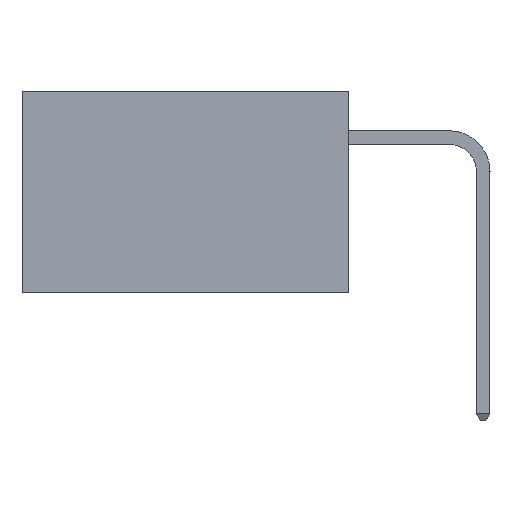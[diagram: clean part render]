
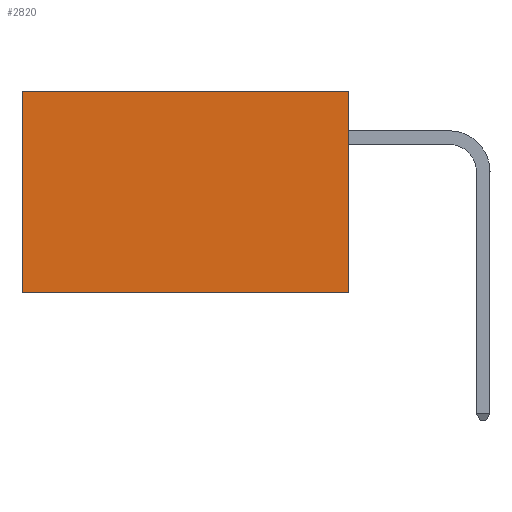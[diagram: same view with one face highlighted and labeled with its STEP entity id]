
A CAD part, left-side view. The second image highlights one B-rep face of the part: STEP entity #2820.
In plain terms, the highlighted planar face has unit normal (-1, 0, 0).
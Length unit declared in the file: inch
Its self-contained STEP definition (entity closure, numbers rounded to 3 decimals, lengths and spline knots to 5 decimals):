
#102 = DIRECTION ( 'NONE',  ( 0., 0., -1. ) ) ;
#106 = DIRECTION ( 'NONE',  ( 1., 0., 0. ) ) ;
#132 = CARTESIAN_POINT ( 'NONE',  ( 0.2875, 0., 0. ) ) ;
#206 = PLANE ( 'NONE',  #11907 ) ;
#261 = ORIENTED_EDGE ( 'NONE', *, *, #8044, .F. ) ;
#651 = CARTESIAN_POINT ( 'NONE',  ( 0.2875, 0., -0.37 ) ) ;
#794 = VECTOR ( 'NONE', #5014, 39.37008 ) ;
#1060 = CARTESIAN_POINT ( 'NONE',  ( 0.2875, 0., 0. ) ) ;
#1378 = CARTESIAN_POINT ( 'NONE',  ( 0.2875, 0., 0. ) ) ;
#1507 = ORIENTED_EDGE ( 'NONE', *, *, #5103, .F. ) ;
#2678 = LINE ( 'NONE', #10681, #14231 ) ;
#2820 = ADVANCED_FACE ( 'NONE', ( #4681 ), #206, .F. ) ;
#4428 = LINE ( 'NONE', #651, #794 ) ;
#4652 = VERTEX_POINT ( 'NONE', #6866 ) ;
#4681 = FACE_OUTER_BOUND ( 'NONE', #7970, .T. ) ;
#4703 = CARTESIAN_POINT ( 'NONE',  ( 0.2875, 0.6, -0.37 ) ) ;
#5014 = DIRECTION ( 'NONE',  ( 0., 1., 0. ) ) ;
#5103 = EDGE_CURVE ( 'NONE', #10782, #11506, #4428, .T. ) ;
#5177 = DIRECTION ( 'NONE',  ( 0., 0., -1. ) ) ;
#5196 = VERTEX_POINT ( 'NONE', #1060 ) ;
#6180 = DIRECTION ( 'NONE',  ( 0., 1., 0. ) ) ;
#6442 = DIRECTION ( 'NONE',  ( 0., 0., -1. ) ) ;
#6866 = CARTESIAN_POINT ( 'NONE',  ( 0.2875, 0.6, 0. ) ) ;
#7374 = ORIENTED_EDGE ( 'NONE', *, *, #10462, .T. ) ;
#7970 = EDGE_LOOP ( 'NONE', ( #11912, #1507, #261, #7374 ) ) ;
#8044 = EDGE_CURVE ( 'NONE', #5196, #10782, #2678, .T. ) ;
#8862 = VECTOR ( 'NONE', #6442, 39.37008 ) ;
#8955 = CARTESIAN_POINT ( 'NONE',  ( 0.2875, 0., -0.37 ) ) ;
#9344 = VECTOR ( 'NONE', #6180, 39.37008 ) ;
#9688 = LINE ( 'NONE', #1378, #9344 ) ;
#9856 = EDGE_CURVE ( 'NONE', #4652, #11506, #11783, .T. ) ;
#10462 = EDGE_CURVE ( 'NONE', #5196, #4652, #9688, .T. ) ;
#10681 = CARTESIAN_POINT ( 'NONE',  ( 0.2875, 0., 0. ) ) ;
#10782 = VERTEX_POINT ( 'NONE', #8955 ) ;
#11506 = VERTEX_POINT ( 'NONE', #4703 ) ;
#11783 = LINE ( 'NONE', #13018, #8862 ) ;
#11907 = AXIS2_PLACEMENT_3D ( 'NONE', #132, #106, #102 ) ;
#11912 = ORIENTED_EDGE ( 'NONE', *, *, #9856, .T. ) ;
#13018 = CARTESIAN_POINT ( 'NONE',  ( 0.2875, 0.6, 0. ) ) ;
#14231 = VECTOR ( 'NONE', #5177, 39.37008 ) ;
